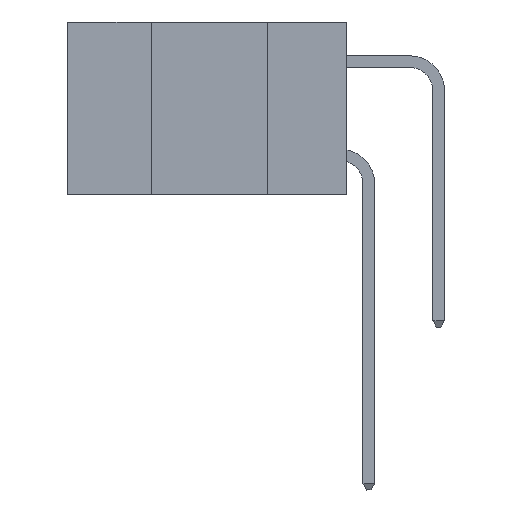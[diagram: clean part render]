
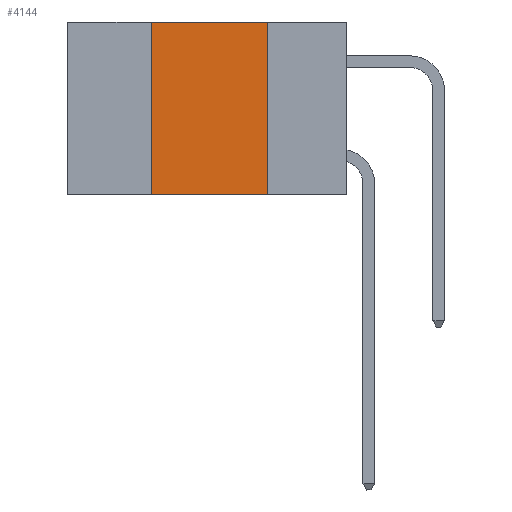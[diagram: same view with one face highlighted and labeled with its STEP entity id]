
A CAD part, left-side view. The second image highlights one B-rep face of the part: STEP entity #4144.
In plain terms, the highlighted planar face has unit normal (-1, 0, 0).
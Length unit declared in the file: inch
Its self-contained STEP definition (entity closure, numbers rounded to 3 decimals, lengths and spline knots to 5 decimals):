
#1013 = VECTOR ( 'NONE', #32025, 39.37008 ) ;
#1748 = ORIENTED_EDGE ( 'NONE', *, *, #5194, .F. ) ;
#4144 = ADVANCED_FACE ( 'NONE', ( #10705 ), #24252, .F. ) ;
#4962 = CARTESIAN_POINT ( 'NONE',  ( 0., 0.42, -0.37 ) ) ;
#5120 = EDGE_CURVE ( 'NONE', #21516, #8833, #20631, .T. ) ;
#5194 = EDGE_CURVE ( 'NONE', #8833, #27919, #30661, .T. ) ;
#8833 = VERTEX_POINT ( 'NONE', #10510 ) ;
#10225 = ORIENTED_EDGE ( 'NONE', *, *, #5120, .F. ) ;
#10510 = CARTESIAN_POINT ( 'NONE',  ( 0., 0.17, 0. ) ) ;
#10546 = DIRECTION ( 'NONE',  ( 1., 0., 0. ) ) ;
#10705 = FACE_OUTER_BOUND ( 'NONE', #34541, .T. ) ;
#13260 = ORIENTED_EDGE ( 'NONE', *, *, #27791, .F. ) ;
#13314 = DIRECTION ( 'NONE',  ( 0., 0., -1. ) ) ;
#14561 = DIRECTION ( 'NONE',  ( 0., -1., 0. ) ) ;
#16637 = ORIENTED_EDGE ( 'NONE', *, *, #27305, .T. ) ;
#18908 = CARTESIAN_POINT ( 'NONE',  ( 0., 0.42, 0. ) ) ;
#19983 = CARTESIAN_POINT ( 'NONE',  ( 0., 0.17, -0.37 ) ) ;
#20133 = LINE ( 'NONE', #18908, #27978 ) ;
#20579 = VECTOR ( 'NONE', #14561, 39.37008 ) ;
#20631 = LINE ( 'NONE', #34089, #21919 ) ;
#21468 = LINE ( 'NONE', #22696, #20579 ) ;
#21516 = VERTEX_POINT ( 'NONE', #29428 ) ;
#21919 = VECTOR ( 'NONE', #29112, 39.37008 ) ;
#22696 = CARTESIAN_POINT ( 'NONE',  ( 0., 0.6, -0.37 ) ) ;
#24252 = PLANE ( 'NONE',  #27390 ) ;
#27078 = CARTESIAN_POINT ( 'NONE',  ( 0., 0.17, 0. ) ) ;
#27305 = EDGE_CURVE ( 'NONE', #35549, #27919, #21468, .T. ) ;
#27390 = AXIS2_PLACEMENT_3D ( 'NONE', #32647, #10546, #13314 ) ;
#27791 = EDGE_CURVE ( 'NONE', #35549, #21516, #20133, .T. ) ;
#27919 = VERTEX_POINT ( 'NONE', #19983 ) ;
#27978 = VECTOR ( 'NONE', #33032, 39.37008 ) ;
#29112 = DIRECTION ( 'NONE',  ( 0., -1., 0. ) ) ;
#29428 = CARTESIAN_POINT ( 'NONE',  ( 0., 0.42, 0. ) ) ;
#30661 = LINE ( 'NONE', #27078, #1013 ) ;
#32025 = DIRECTION ( 'NONE',  ( 0., 0., -1. ) ) ;
#32647 = CARTESIAN_POINT ( 'NONE',  ( 0., 0.6, 0. ) ) ;
#33032 = DIRECTION ( 'NONE',  ( 0., 0., 1. ) ) ;
#34089 = CARTESIAN_POINT ( 'NONE',  ( 0., 0.6, 0. ) ) ;
#34541 = EDGE_LOOP ( 'NONE', ( #1748, #10225, #13260, #16637 ) ) ;
#35549 = VERTEX_POINT ( 'NONE', #4962 ) ;
